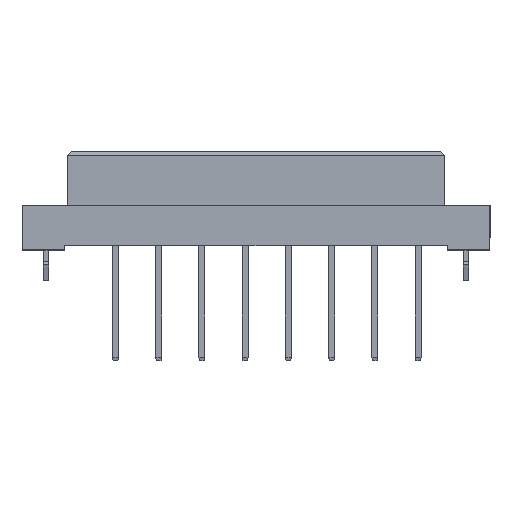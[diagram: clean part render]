
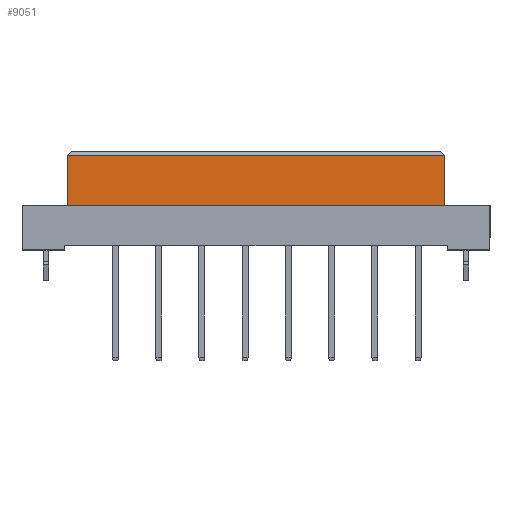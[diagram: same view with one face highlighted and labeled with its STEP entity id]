
A CAD part, top view. The second image highlights one B-rep face of the part: STEP entity #9051.
In plain terms, the highlighted planar face has unit normal (0, 0, 1).
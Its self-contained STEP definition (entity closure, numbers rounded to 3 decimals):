
#904 = CARTESIAN_POINT ( 'NONE',  ( 22.2, -0.5, 4.25 ) ) ;
#2143 = VECTOR ( 'NONE', #11808, 1000. ) ;
#2256 = LINE ( 'NONE', #8699, #4079 ) ;
#2950 = ORIENTED_EDGE ( 'NONE', *, *, #13963, .T. ) ;
#3284 = VERTEX_POINT ( 'NONE', #3708 ) ;
#3490 = VECTOR ( 'NONE', #18166, 1000. ) ;
#3708 = CARTESIAN_POINT ( 'NONE',  ( -22.2, -6.4, 4.25 ) ) ;
#4079 = VECTOR ( 'NONE', #13525, 1000. ) ;
#5306 = CARTESIAN_POINT ( 'NONE',  ( 22.2, -6.4, 4.25 ) ) ;
#5671 = DIRECTION ( 'NONE',  ( 0., 0., 1. ) ) ;
#5928 = ORIENTED_EDGE ( 'NONE', *, *, #10865, .T. ) ;
#6050 = EDGE_CURVE ( 'NONE', #12046, #11789, #2256, .T. ) ;
#6422 = CARTESIAN_POINT ( 'NONE',  ( 22.2, -6.4, 4.25 ) ) ;
#6570 = CARTESIAN_POINT ( 'NONE',  ( 22.2, -6.4, 4.25 ) ) ;
#7601 = VECTOR ( 'NONE', #12964, 1000. ) ;
#8699 = CARTESIAN_POINT ( 'NONE',  ( -22.2, -0.5, 4.25 ) ) ;
#9051 = ADVANCED_FACE ( 'NONE', ( #19106 ), #12433, .T. ) ;
#10281 = ORIENTED_EDGE ( 'NONE', *, *, #6050, .T. ) ;
#10502 = AXIS2_PLACEMENT_3D ( 'NONE', #15771, #5671, #15666 ) ;
#10865 = EDGE_CURVE ( 'NONE', #3284, #17391, #21145, .T. ) ;
#11293 = EDGE_CURVE ( 'NONE', #3284, #11789, #13946, .T. ) ;
#11789 = VERTEX_POINT ( 'NONE', #21136 ) ;
#11808 = DIRECTION ( 'NONE',  ( 0., 1., 0. ) ) ;
#12046 = VERTEX_POINT ( 'NONE', #904 ) ;
#12433 = PLANE ( 'NONE',  #10502 ) ;
#12902 = ORIENTED_EDGE ( 'NONE', *, *, #11293, .F. ) ;
#12964 = DIRECTION ( 'NONE',  ( 1., 0., 0. ) ) ;
#13525 = DIRECTION ( 'NONE',  ( -1., 0., 0. ) ) ;
#13946 = LINE ( 'NONE', #15459, #2143 ) ;
#13963 = EDGE_CURVE ( 'NONE', #17391, #12046, #19674, .T. ) ;
#15459 = CARTESIAN_POINT ( 'NONE',  ( -22.2, -6.4, 4.25 ) ) ;
#15666 = DIRECTION ( 'NONE',  ( 1., 0., 0. ) ) ;
#15771 = CARTESIAN_POINT ( 'NONE',  ( 22.2, -6.4, 4.25 ) ) ;
#17391 = VERTEX_POINT ( 'NONE', #5306 ) ;
#18166 = DIRECTION ( 'NONE',  ( 0., 1., 0. ) ) ;
#19106 = FACE_OUTER_BOUND ( 'NONE', #19807, .T. ) ;
#19674 = LINE ( 'NONE', #6570, #3490 ) ;
#19807 = EDGE_LOOP ( 'NONE', ( #2950, #10281, #12902, #5928 ) ) ;
#21136 = CARTESIAN_POINT ( 'NONE',  ( -22.2, -0.5, 4.25 ) ) ;
#21145 = LINE ( 'NONE', #6422, #7601 ) ;
